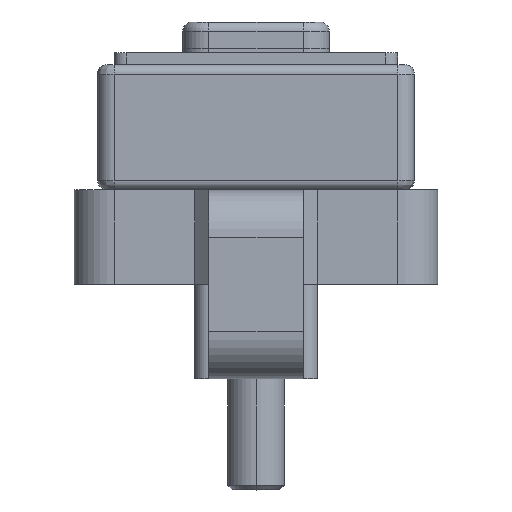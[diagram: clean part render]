
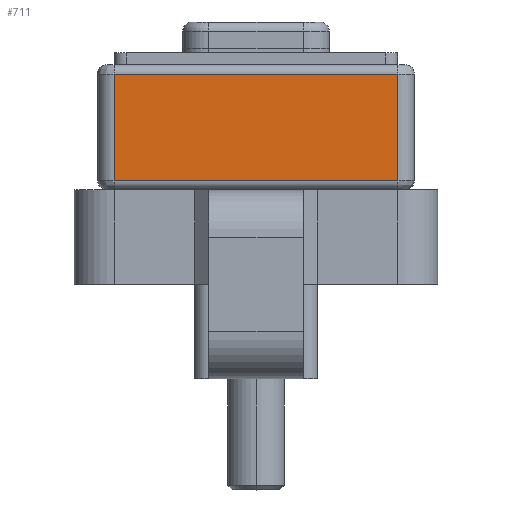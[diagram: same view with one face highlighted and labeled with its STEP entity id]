
A CAD part, left-side view. The second image highlights one B-rep face of the part: STEP entity #711.
In plain terms, the highlighted planar face has unit normal (-1, 0, 0).
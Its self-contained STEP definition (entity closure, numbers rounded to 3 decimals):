
#711 = ADVANCED_FACE ( 'NONE', ( #4337 ), #21000, .F. ) ;
#1168 = DIRECTION ( 'NONE',  ( 0., 0., -1. ) ) ;
#2602 = DIRECTION ( 'NONE',  ( 0., 1., 0. ) ) ;
#4332 = CARTESIAN_POINT ( 'NONE',  ( -6.15, 3., 4.45 ) ) ;
#4337 = FACE_OUTER_BOUND ( 'NONE', #9787, .T. ) ;
#5498 = DIRECTION ( 'NONE',  ( 0., 0., 1. ) ) ;
#5854 = DIRECTION ( 'NONE',  ( 1., 0., 0. ) ) ;
#6054 = LINE ( 'NONE', #9216, #6486 ) ;
#6082 = CARTESIAN_POINT ( 'NONE',  ( -6.15, 0., 3.5 ) ) ;
#6143 = ORIENTED_EDGE ( 'NONE', *, *, #20027, .T. ) ;
#6328 = VERTEX_POINT ( 'NONE', #9644 ) ;
#6486 = VECTOR ( 'NONE', #17703, 1000. ) ;
#7125 = CARTESIAN_POINT ( 'NONE',  ( -6.15, 3., 2.2 ) ) ;
#7227 = EDGE_CURVE ( 'NONE', #20866, #18646, #6054, .T. ) ;
#7437 = LINE ( 'NONE', #15499, #10103 ) ;
#9216 = CARTESIAN_POINT ( 'NONE',  ( -6.15, 3., 2.2 ) ) ;
#9335 = CARTESIAN_POINT ( 'NONE',  ( -6.15, 3., 4.8 ) ) ;
#9644 = CARTESIAN_POINT ( 'NONE',  ( -6.15, -3., 4.45 ) ) ;
#9787 = EDGE_LOOP ( 'NONE', ( #18052, #16747, #19800, #6143 ) ) ;
#10103 = VECTOR ( 'NONE', #14176, 1000. ) ;
#10877 = VERTEX_POINT ( 'NONE', #4332 ) ;
#11783 = EDGE_CURVE ( 'NONE', #6328, #10877, #7437, .T. ) ;
#12033 = CARTESIAN_POINT ( 'NONE',  ( -6.15, -3., 2.2 ) ) ;
#12915 = LINE ( 'NONE', #9335, #16018 ) ;
#13890 = VECTOR ( 'NONE', #5498, 1000. ) ;
#14176 = DIRECTION ( 'NONE',  ( 0., 1., 0. ) ) ;
#15499 = CARTESIAN_POINT ( 'NONE',  ( -6.15, -3., 4.45 ) ) ;
#15638 = AXIS2_PLACEMENT_3D ( 'NONE', #6082, #5854, #2602 ) ;
#15880 = CARTESIAN_POINT ( 'NONE',  ( -6.15, -3., 2.2 ) ) ;
#16018 = VECTOR ( 'NONE', #1168, 1000. ) ;
#16747 = ORIENTED_EDGE ( 'NONE', *, *, #19140, .T. ) ;
#17703 = DIRECTION ( 'NONE',  ( 0., -1., 0. ) ) ;
#18052 = ORIENTED_EDGE ( 'NONE', *, *, #7227, .T. ) ;
#18568 = LINE ( 'NONE', #12033, #13890 ) ;
#18646 = VERTEX_POINT ( 'NONE', #15880 ) ;
#19140 = EDGE_CURVE ( 'NONE', #18646, #6328, #18568, .T. ) ;
#19800 = ORIENTED_EDGE ( 'NONE', *, *, #11783, .T. ) ;
#20027 = EDGE_CURVE ( 'NONE', #10877, #20866, #12915, .T. ) ;
#20866 = VERTEX_POINT ( 'NONE', #7125 ) ;
#21000 = PLANE ( 'NONE',  #15638 ) ;
